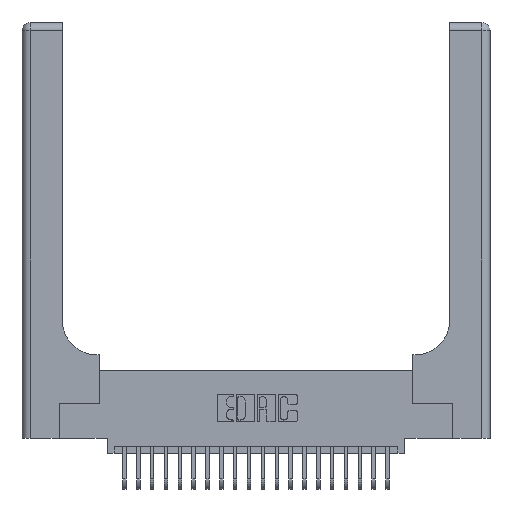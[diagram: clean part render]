
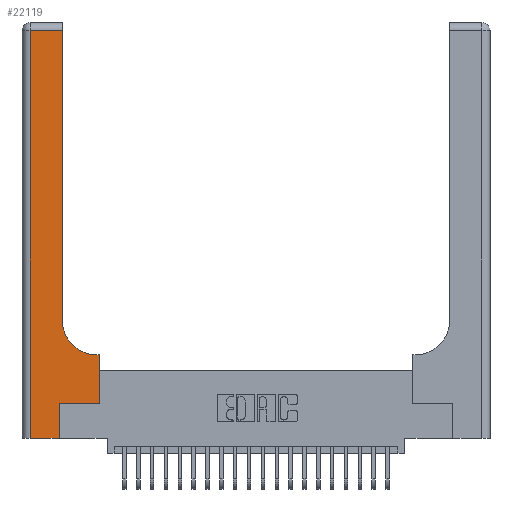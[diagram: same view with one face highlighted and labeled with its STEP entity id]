
A CAD part, top view. The second image highlights one B-rep face of the part: STEP entity #22119.
In plain terms, the highlighted planar face has unit normal (0, 0, 1).
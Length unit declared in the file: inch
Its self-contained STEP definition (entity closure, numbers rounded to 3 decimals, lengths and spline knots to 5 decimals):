
#247 = ORIENTED_EDGE ( 'NONE', *, *, #15347, .T. ) ;
#366 = DIRECTION ( 'NONE',  ( 0., 1., 0. ) ) ;
#473 = DIRECTION ( 'NONE',  ( -1., 0., 0. ) ) ;
#521 = CARTESIAN_POINT ( 'NONE',  ( 0.5415, 0.85, 0.37 ) ) ;
#543 = EDGE_CURVE ( 'NONE', #4032, #2558, #7176, .T. ) ;
#559 = LINE ( 'NONE', #18931, #20930 ) ;
#2015 = ORIENTED_EDGE ( 'NONE', *, *, #3551, .T. ) ;
#2515 = DIRECTION ( 'NONE',  ( 1., 0., 0. ) ) ;
#2558 = VERTEX_POINT ( 'NONE', #5112 ) ;
#3551 = EDGE_CURVE ( 'NONE', #13622, #9833, #12105, .T. ) ;
#3934 = DIRECTION ( 'NONE',  ( 1., 0., 0. ) ) ;
#4021 = DIRECTION ( 'NONE',  ( -1., 0., 0. ) ) ;
#4032 = VERTEX_POINT ( 'NONE', #15408 ) ;
#4330 = EDGE_CURVE ( 'NONE', #16050, #21684, #4656, .T. ) ;
#4656 = LINE ( 'NONE', #22234, #25078 ) ;
#4845 = EDGE_CURVE ( 'NONE', #21684, #8222, #7994, .T. ) ;
#5112 = CARTESIAN_POINT ( 'NONE',  ( 0.2915, 2.94, 0.37 ) ) ;
#6564 = CARTESIAN_POINT ( 'NONE',  ( 0., 0., 0.37 ) ) ;
#6568 = VECTOR ( 'NONE', #366, 39.37008 ) ;
#7052 = VECTOR ( 'NONE', #473, 39.37008 ) ;
#7176 = LINE ( 'NONE', #22369, #18655 ) ;
#7546 = CARTESIAN_POINT ( 'NONE',  ( 0.269, 0., 0.37 ) ) ;
#7900 = CARTESIAN_POINT ( 'NONE',  ( 0.5415, 0.6, 0.37 ) ) ;
#7994 = LINE ( 'NONE', #6564, #14753 ) ;
#8222 = VERTEX_POINT ( 'NONE', #7546 ) ;
#8975 = ORIENTED_EDGE ( 'NONE', *, *, #543, .T. ) ;
#9058 = DIRECTION ( 'NONE',  ( 1., 0., 0. ) ) ;
#9174 = DIRECTION ( 'NONE',  ( 0., 1., 0. ) ) ;
#9460 = CARTESIAN_POINT ( 'NONE',  ( 0.5585, 0.6, 0.37 ) ) ;
#9833 = VERTEX_POINT ( 'NONE', #7900 ) ;
#10044 = DIRECTION ( 'NONE',  ( 0., 0., -1. ) ) ;
#10219 = EDGE_CURVE ( 'NONE', #8222, #12465, #22023, .T. ) ;
#10432 = CARTESIAN_POINT ( 'NONE',  ( 0.269, 0.25, 0.37 ) ) ;
#10457 = ORIENTED_EDGE ( 'NONE', *, *, #17090, .T. ) ;
#10519 = DIRECTION ( 'NONE',  ( 0., 1., 0. ) ) ;
#10659 = CARTESIAN_POINT ( 'NONE',  ( 0.2915, 0.6, 0.37 ) ) ;
#11105 = ORIENTED_EDGE ( 'NONE', *, *, #13944, .T. ) ;
#11305 = ORIENTED_EDGE ( 'NONE', *, *, #4330, .T. ) ;
#11976 = FACE_OUTER_BOUND ( 'NONE', #13816, .T. ) ;
#12105 = LINE ( 'NONE', #10659, #25432 ) ;
#12465 = VERTEX_POINT ( 'NONE', #10432 ) ;
#12919 = CIRCLE ( 'NONE', #13640, 0.25 ) ;
#13622 = VERTEX_POINT ( 'NONE', #9460 ) ;
#13640 = AXIS2_PLACEMENT_3D ( 'NONE', #521, #14296, #2515 ) ;
#13816 = EDGE_LOOP ( 'NONE', ( #8975, #20320, #11305, #21861, #21128, #11105, #10457, #2015, #247 ) ) ;
#13944 = EDGE_CURVE ( 'NONE', #12465, #21880, #559, .T. ) ;
#14296 = DIRECTION ( 'NONE',  ( 0., 0., -1. ) ) ;
#14335 = DIRECTION ( 'NONE',  ( -1., 0., 0. ) ) ;
#14753 = VECTOR ( 'NONE', #3934, 39.37008 ) ;
#14986 = VECTOR ( 'NONE', #9174, 39.37008 ) ;
#15347 = EDGE_CURVE ( 'NONE', #9833, #4032, #12919, .T. ) ;
#15408 = CARTESIAN_POINT ( 'NONE',  ( 0.2915, 0.85, 0.37 ) ) ;
#16050 = VERTEX_POINT ( 'NONE', #16272 ) ;
#16056 = EDGE_CURVE ( 'NONE', #2558, #16050, #22841, .T. ) ;
#16232 = DIRECTION ( 'NONE',  ( 0., -1., 0. ) ) ;
#16272 = CARTESIAN_POINT ( 'NONE',  ( 0.06, 2.94, 0.37 ) ) ;
#16780 = CARTESIAN_POINT ( 'NONE',  ( 0.5585, 0.25, 0.37 ) ) ;
#16859 = CARTESIAN_POINT ( 'NONE',  ( 0.269, 0., 0.37 ) ) ;
#17090 = EDGE_CURVE ( 'NONE', #21880, #13622, #25612, .T. ) ;
#18655 = VECTOR ( 'NONE', #10519, 39.37008 ) ;
#18931 = CARTESIAN_POINT ( 'NONE',  ( 0.269, 0.25, 0.37 ) ) ;
#19738 = CARTESIAN_POINT ( 'NONE',  ( 0., 3., 0.37 ) ) ;
#20320 = ORIENTED_EDGE ( 'NONE', *, *, #16056, .T. ) ;
#20930 = VECTOR ( 'NONE', #9058, 39.37008 ) ;
#21128 = ORIENTED_EDGE ( 'NONE', *, *, #10219, .T. ) ;
#21684 = VERTEX_POINT ( 'NONE', #22354 ) ;
#21861 = ORIENTED_EDGE ( 'NONE', *, *, #4845, .T. ) ;
#21880 = VERTEX_POINT ( 'NONE', #16780 ) ;
#21976 = PLANE ( 'NONE',  #22874 ) ;
#22023 = LINE ( 'NONE', #16859, #6568 ) ;
#22119 = ADVANCED_FACE ( 'NONE', ( #11976 ), #21976, .F. ) ;
#22234 = CARTESIAN_POINT ( 'NONE',  ( 0.06, 3., 0.37 ) ) ;
#22354 = CARTESIAN_POINT ( 'NONE',  ( 0.06, 0., 0.37 ) ) ;
#22369 = CARTESIAN_POINT ( 'NONE',  ( 0.2915, 3., 0.37 ) ) ;
#22776 = CARTESIAN_POINT ( 'NONE',  ( 0.5585, 0.25, 0.37 ) ) ;
#22841 = LINE ( 'NONE', #23727, #7052 ) ;
#22874 = AXIS2_PLACEMENT_3D ( 'NONE', #19738, #10044, #4021 ) ;
#23727 = CARTESIAN_POINT ( 'NONE',  ( 0., 2.94, 0.37 ) ) ;
#25078 = VECTOR ( 'NONE', #16232, 39.37008 ) ;
#25432 = VECTOR ( 'NONE', #14335, 39.37008 ) ;
#25612 = LINE ( 'NONE', #22776, #14986 ) ;
